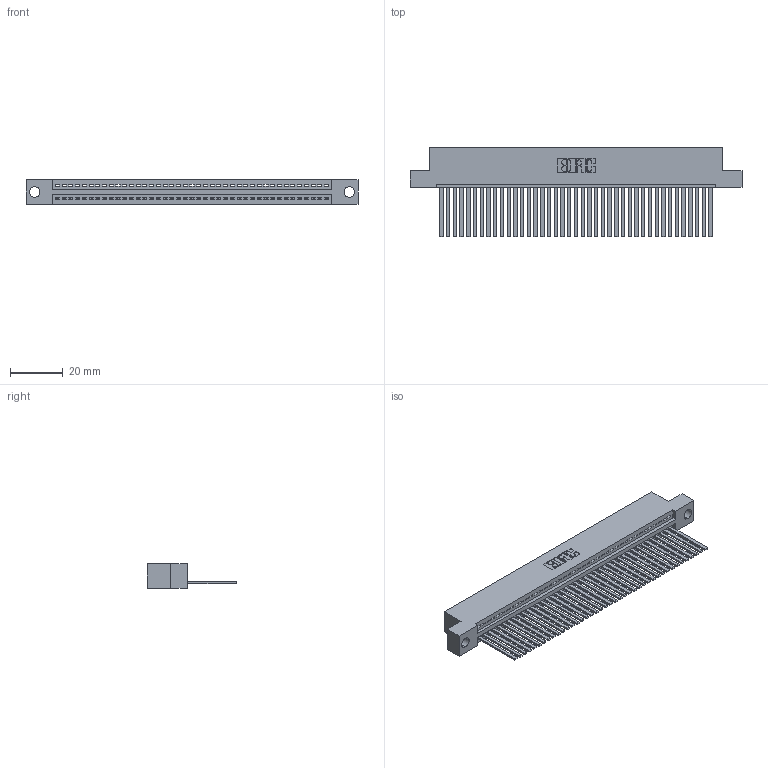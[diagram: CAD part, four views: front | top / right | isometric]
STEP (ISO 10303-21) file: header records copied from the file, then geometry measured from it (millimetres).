
FILE_DESCRIPTION (( 'STEP AP203' ), '1' );
FILE_NAME ('395-041-544-104.STEP', '2019-10-22T11:07:28', ( '' ), ( '' ), 'SwSTEP 2.0', 'SolidWorks 2016', '' );
FILE_SCHEMA (( 'CONFIG_CONTROL_DESIGN' ));
Length unit declared in the file: inch
Products named in the file (3): 395-041-544-104; 345 Part_Flush Mounting Lugs - 0.156 Dia-TH; 345-292-001_345-293-144
Assembly tree (42 placements, depth 2):
  395-041-544-104
    345 Part_Flush Mounting Lugs - 0.156 Dia-TH
    345-292-001_345-293-144  x41
Bounding box: 125.35 x 33.96 x 9.4 mm (x, y, z)
Volume: 12284.6 mm3; surface area: 17545.7 mm2
Topology: 42 solids, 42 shells, 2258 faces, 6819 edges, 4490 vertices
Faces by surface type: plane 1556, cylinder 702
Entity records: 30811 total; most frequent: CARTESIAN_POINT 5343, ORIENTED_EDGE 5318, DIRECTION 4665, EDGE_CURVE 2659, VECTOR 2367, LINE 2367, VERTEX_POINT 1770, AXIS2_PLACEMENT_3D 1149
